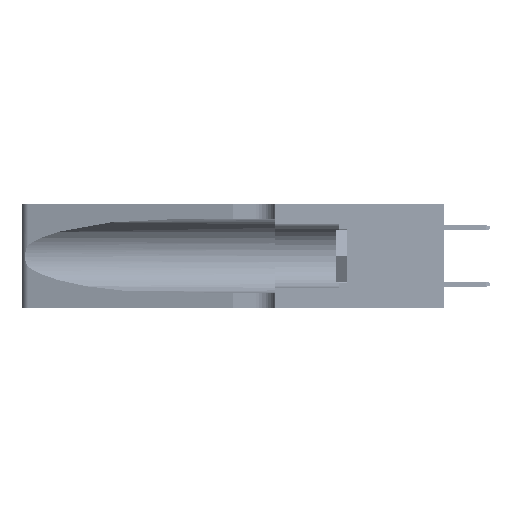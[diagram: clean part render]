
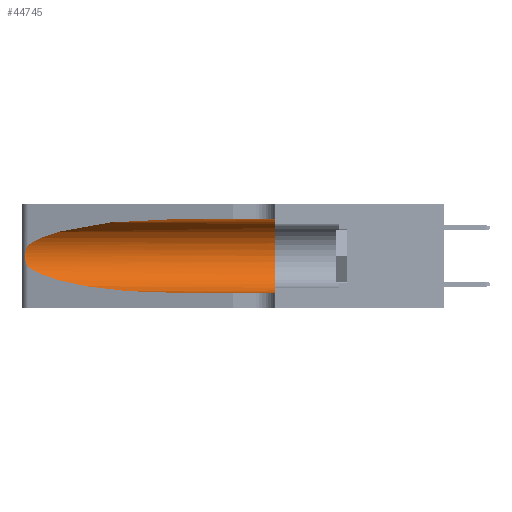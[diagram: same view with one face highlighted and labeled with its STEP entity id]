
A CAD part, left-side view. The second image highlights one B-rep face of the part: STEP entity #44745.
In plain terms, the highlighted cylindrical face has radius 3.308 mm (diameter 6.617 mm), a partial arc.
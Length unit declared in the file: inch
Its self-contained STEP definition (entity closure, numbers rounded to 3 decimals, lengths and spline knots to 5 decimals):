
#2052 = LINE ( 'NONE', #49368, #10328 ) ;
#3057 = B_SPLINE_CURVE_WITH_KNOTS ( 'NONE', 3,
 ( #3791, #27915, #40003, #15974, #44030, #20029, #48070, #24051, #52094, #28090, #3955, #32129, #8061, #36147 ),
 .UNSPECIFIED., .F., .F.,
 ( 4, 2, 2, 2, 2, 2, 4 ),
 ( 0., 0.00027, 0.00053, 0.00107, 0.0016, 0.00187, 0.00214 ),
 .UNSPECIFIED. ) ;
#3791 = CARTESIAN_POINT ( 'NONE',  ( 0.25487, 1.22718, 0.22369 ) ) ;
#3955 = CARTESIAN_POINT ( 'NONE',  ( 0.25789, 1.23486, 0.15765 ) ) ;
#4099 = CARTESIAN_POINT ( 'NONE',  ( 0.2373, 1.15595, 0.08982 ) ) ;
#4278 = CARTESIAN_POINT ( 'NONE',  ( 0.18966, 0.96281, 0.05475 ) ) ;
#7058 = DIRECTION ( 'NONE',  ( 0., -1., 0. ) ) ;
#8061 = CARTESIAN_POINT ( 'NONE',  ( 0.25555, 1.22993, 0.14849 ) ) ;
#8200 = CARTESIAN_POINT ( 'NONE',  ( 0.25487, 1.22718, 0.14631 ) ) ;
#9238 = CARTESIAN_POINT ( 'NONE',  ( 0.25487, 1.22718, 0.22369 ) ) ;
#10328 = VECTOR ( 'NONE', #20988, 39.37008 ) ;
#11143 = ORIENTED_EDGE ( 'NONE', *, *, #22056, .T. ) ;
#11819 = CYLINDRICAL_SURFACE ( 'NONE', #20691, 0.13025 ) ;
#12985 = DIRECTION ( 'NONE',  ( 0., -1., 0. ) ) ;
#13082 = ORIENTED_EDGE ( 'NONE', *, *, #26380, .T. ) ;
#13095 = FACE_OUTER_BOUND ( 'NONE', #51623, .T. ) ;
#15162 = EDGE_CURVE ( 'NONE', #16319, #38721, #45483, .T. ) ;
#15974 = CARTESIAN_POINT ( 'NONE',  ( 0.25787, 1.23484, 0.2124 ) ) ;
#16319 = VERTEX_POINT ( 'NONE', #51175 ) ;
#18866 = CARTESIAN_POINT ( 'NONE',  ( 0.1305, 0.72297, 0.31525 ) ) ;
#19883 = CARTESIAN_POINT ( 'NONE',  ( 0.25487, 1.22718, 0.14631 ) ) ;
#20029 = CARTESIAN_POINT ( 'NONE',  ( 0.26018, 1.23835, 0.19895 ) ) ;
#20691 = AXIS2_PLACEMENT_3D ( 'NONE', #25080, #12985, #49080 ) ;
#20973 = AXIS2_PLACEMENT_3D ( 'NONE', #22943, #50976, #26989 ) ;
#20988 = DIRECTION ( 'NONE',  ( 0., -1., 0. ) ) ;
#21540 = CARTESIAN_POINT ( 'NONE',  ( 0.1305, 0.35, 0.05475 ) ) ;
#22056 = EDGE_CURVE ( 'NONE', #47078, #49842, #40470, .T. ) ;
#22869 = CARTESIAN_POINT ( 'NONE',  ( 0.25487, 1.22718, 0.22369 ) ) ;
#22943 = CARTESIAN_POINT ( 'NONE',  ( 0.1305, 0.35, 0.185 ) ) ;
#24051 = CARTESIAN_POINT ( 'NONE',  ( 0.26075, 1.23896, 0.178 ) ) ;
#24158 = VECTOR ( 'NONE', #7058, 39.37008 ) ;
#25080 = CARTESIAN_POINT ( 'NONE',  ( 0.1305, 1.61858, 0.185 ) ) ;
#25561 = VERTEX_POINT ( 'NONE', #19883 ) ;
#26380 = EDGE_CURVE ( 'NONE', #25561, #16319, #31155, .T. ) ;
#26860 = ORIENTED_EDGE ( 'NONE', *, *, #41039, .T. ) ;
#26989 = DIRECTION ( 'NONE',  ( 0., 0., 1. ) ) ;
#27915 = CARTESIAN_POINT ( 'NONE',  ( 0.25555, 1.22994, 0.2215 ) ) ;
#28090 = CARTESIAN_POINT ( 'NONE',  ( 0.25856, 1.23593, 0.16098 ) ) ;
#30776 = CARTESIAN_POINT ( 'NONE',  ( 0.2373, 1.15595, 0.28018 ) ) ;
#31155 =( BOUNDED_CURVE ( )  B_SPLINE_CURVE ( 3, ( #8200, #4099, #4278, #32434 ),
 .UNSPECIFIED., .F., .F. ) 
 B_SPLINE_CURVE_WITH_KNOTS ( ( 4, 4 ),
 ( 3.44316, 4.71239 ),
 .UNSPECIFIED. ) 
 CURVE ( )  GEOMETRIC_REPRESENTATION_ITEM ( )  RATIONAL_B_SPLINE_CURVE ( ( 1., 0.87, 0.87, 1. ) ) 
 REPRESENTATION_ITEM ( '' )  );
#32129 = CARTESIAN_POINT ( 'NONE',  ( 0.25639, 1.23186, 0.15144 ) ) ;
#32309 = VERTEX_POINT ( 'NONE', #37748 ) ;
#32434 = CARTESIAN_POINT ( 'NONE',  ( 0.1305, 0.72297, 0.05475 ) ) ;
#34022 = CARTESIAN_POINT ( 'NONE',  ( 0.1305, 0.72297, 0.31525 ) ) ;
#35646 = ORIENTED_EDGE ( 'NONE', *, *, #49563, .F. ) ;
#36147 = CARTESIAN_POINT ( 'NONE',  ( 0.25487, 1.22718, 0.14631 ) ) ;
#37748 = CARTESIAN_POINT ( 'NONE',  ( 0.1305, 0.35, 0.31525 ) ) ;
#38163 = ORIENTED_EDGE ( 'NONE', *, *, #51074, .F. ) ;
#38721 = VERTEX_POINT ( 'NONE', #21540 ) ;
#40003 = CARTESIAN_POINT ( 'NONE',  ( 0.25639, 1.23184, 0.21858 ) ) ;
#40470 =( BOUNDED_CURVE ( )  B_SPLINE_CURVE ( 3, ( #18866, #50742, #30776, #22869 ),
 .UNSPECIFIED., .F., .T. ) 
 B_SPLINE_CURVE_WITH_KNOTS ( ( 4, 4 ),
 ( 1.5708, 2.84003 ),
 .UNSPECIFIED. ) 
 CURVE ( )  GEOMETRIC_REPRESENTATION_ITEM ( )  RATIONAL_B_SPLINE_CURVE ( ( 1., 0.87, 0.87, 1. ) ) 
 REPRESENTATION_ITEM ( '' )  );
#41039 = EDGE_CURVE ( 'NONE', #49842, #25561, #3057, .T. ) ;
#42516 = CARTESIAN_POINT ( 'NONE',  ( 0.1305, 1.61858, 0.05475 ) ) ;
#44030 = CARTESIAN_POINT ( 'NONE',  ( 0.25854, 1.2359, 0.20912 ) ) ;
#44745 = ADVANCED_FACE ( 'NONE', ( #13095 ), #11819, .F. ) ;
#45057 = ORIENTED_EDGE ( 'NONE', *, *, #15162, .T. ) ;
#45483 = LINE ( 'NONE', #42516, #24158 ) ;
#47078 = VERTEX_POINT ( 'NONE', #34022 ) ;
#48070 = CARTESIAN_POINT ( 'NONE',  ( 0.26075, 1.23896, 0.19203 ) ) ;
#49011 = CIRCLE ( 'NONE', #20973, 0.13025 ) ;
#49080 = DIRECTION ( 'NONE',  ( 0., 0., -1. ) ) ;
#49368 = CARTESIAN_POINT ( 'NONE',  ( 0.1305, 1.61858, 0.31525 ) ) ;
#49563 = EDGE_CURVE ( 'NONE', #32309, #38721, #49011, .T. ) ;
#49842 = VERTEX_POINT ( 'NONE', #9238 ) ;
#50742 = CARTESIAN_POINT ( 'NONE',  ( 0.18966, 0.96281, 0.31525 ) ) ;
#50976 = DIRECTION ( 'NONE',  ( 0., 1., 0. ) ) ;
#51074 = EDGE_CURVE ( 'NONE', #47078, #32309, #2052, .T. ) ;
#51175 = CARTESIAN_POINT ( 'NONE',  ( 0.1305, 0.72297, 0.05475 ) ) ;
#51623 = EDGE_LOOP ( 'NONE', ( #11143, #26860, #13082, #45057, #35646, #38163 ) ) ;
#52094 = CARTESIAN_POINT ( 'NONE',  ( 0.26017, 1.23833, 0.17102 ) ) ;
